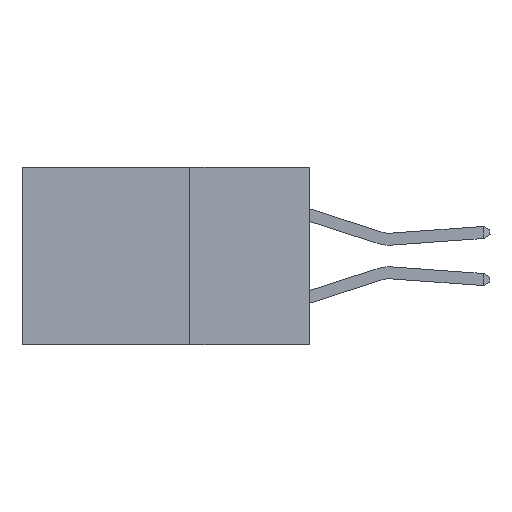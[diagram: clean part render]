
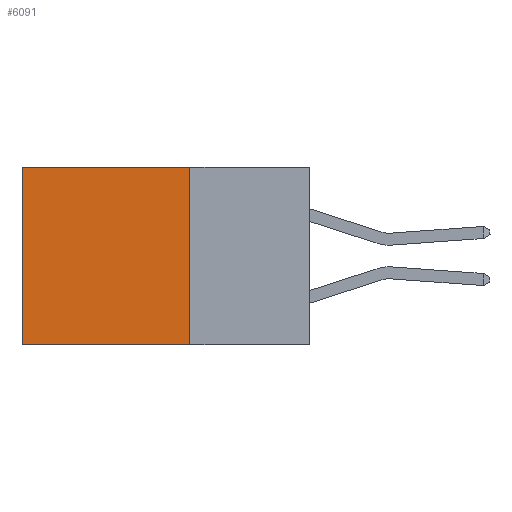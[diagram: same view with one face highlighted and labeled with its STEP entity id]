
A CAD part, left-side view. The second image highlights one B-rep face of the part: STEP entity #6091.
In plain terms, the highlighted planar face has unit normal (-1, 0, 0).
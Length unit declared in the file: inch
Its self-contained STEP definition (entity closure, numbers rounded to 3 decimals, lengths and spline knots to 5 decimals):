
#191 = ORIENTED_EDGE ( 'NONE', *, *, #1929, .T. ) ;
#793 = EDGE_CURVE ( 'NONE', #1340, #1767, #5571, .T. ) ;
#1340 = VERTEX_POINT ( 'NONE', #6257 ) ;
#1508 = EDGE_CURVE ( 'NONE', #1767, #9747, #7310, .T. ) ;
#1767 = VERTEX_POINT ( 'NONE', #5826 ) ;
#1929 = EDGE_CURVE ( 'NONE', #3867, #9747, #10091, .T. ) ;
#2470 = CARTESIAN_POINT ( 'NONE',  ( 0.2615, 0.6, 0. ) ) ;
#3027 = ORIENTED_EDGE ( 'NONE', *, *, #793, .F. ) ;
#3867 = VERTEX_POINT ( 'NONE', #2470 ) ;
#4307 = PLANE ( 'NONE',  #7374 ) ;
#4342 = DIRECTION ( 'NONE',  ( 1., 0., 0. ) ) ;
#4585 = DIRECTION ( 'NONE',  ( 0., 0., -1. ) ) ;
#5105 = CARTESIAN_POINT ( 'NONE',  ( 0.2615, 0.6, -0.37 ) ) ;
#5299 = ORIENTED_EDGE ( 'NONE', *, *, #5403, .T. ) ;
#5403 = EDGE_CURVE ( 'NONE', #1340, #3867, #6619, .T. ) ;
#5440 = EDGE_LOOP ( 'NONE', ( #191, #6924, #3027, #5299 ) ) ;
#5494 = DIRECTION ( 'NONE',  ( 0., 1., 0. ) ) ;
#5571 = LINE ( 'NONE', #8363, #5835 ) ;
#5826 = CARTESIAN_POINT ( 'NONE',  ( 0.2615, 0.25, -0.37 ) ) ;
#5835 = VECTOR ( 'NONE', #8362, 39.37008 ) ;
#5960 = DIRECTION ( 'NONE',  ( 0., 1., 0. ) ) ;
#6038 = CARTESIAN_POINT ( 'NONE',  ( 0.2615, 0.6, -0.37 ) ) ;
#6091 = ADVANCED_FACE ( 'NONE', ( #8082 ), #4307, .F. ) ;
#6118 = CARTESIAN_POINT ( 'NONE',  ( 0.2615, 0.25, -0.37 ) ) ;
#6257 = CARTESIAN_POINT ( 'NONE',  ( 0.2615, 0.25, 0. ) ) ;
#6387 = VECTOR ( 'NONE', #5960, 39.37008 ) ;
#6619 = LINE ( 'NONE', #9086, #6387 ) ;
#6924 = ORIENTED_EDGE ( 'NONE', *, *, #1508, .F. ) ;
#7060 = VECTOR ( 'NONE', #5494, 39.37008 ) ;
#7310 = LINE ( 'NONE', #6118, #7060 ) ;
#7374 = AXIS2_PLACEMENT_3D ( 'NONE', #9074, #4342, #9861 ) ;
#7804 = VECTOR ( 'NONE', #4585, 39.37008 ) ;
#8082 = FACE_OUTER_BOUND ( 'NONE', #5440, .T. ) ;
#8362 = DIRECTION ( 'NONE',  ( 0., 0., -1. ) ) ;
#8363 = CARTESIAN_POINT ( 'NONE',  ( 0.2615, 0.25, -0.37 ) ) ;
#9074 = CARTESIAN_POINT ( 'NONE',  ( 0.2615, 0.25, -0.37 ) ) ;
#9086 = CARTESIAN_POINT ( 'NONE',  ( 0.2615, 0.25, 0. ) ) ;
#9747 = VERTEX_POINT ( 'NONE', #6038 ) ;
#9861 = DIRECTION ( 'NONE',  ( 0., 0., -1. ) ) ;
#10091 = LINE ( 'NONE', #5105, #7804 ) ;
